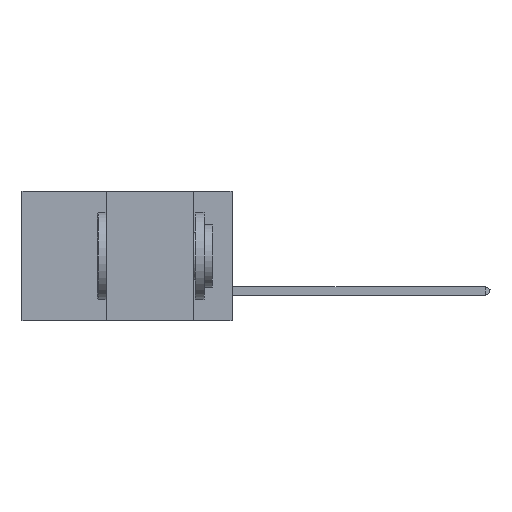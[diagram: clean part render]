
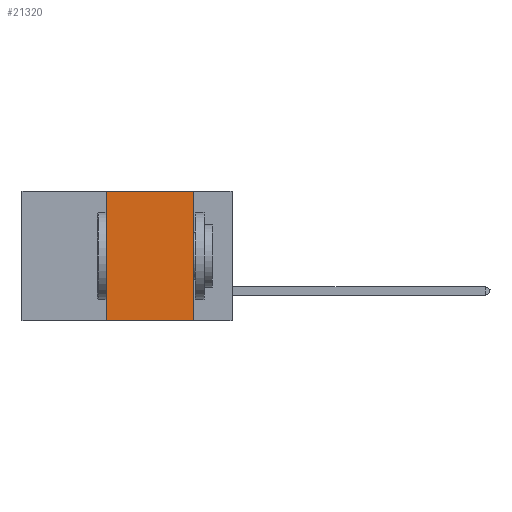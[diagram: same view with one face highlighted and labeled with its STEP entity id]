
A CAD part, left-side view. The second image highlights one B-rep face of the part: STEP entity #21320.
In plain terms, the highlighted planar face has unit normal (-1, 0, 0).
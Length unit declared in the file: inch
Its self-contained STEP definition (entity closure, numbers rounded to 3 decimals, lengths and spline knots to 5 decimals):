
#302 = VERTEX_POINT ( 'NONE', #35650 ) ;
#1284 = DIRECTION ( 'NONE',  ( 0., 0., -1. ) ) ;
#1719 = CARTESIAN_POINT ( 'NONE',  ( 0., 0.6, 0. ) ) ;
#3242 = CARTESIAN_POINT ( 'NONE',  ( 0., 0.36, 0. ) ) ;
#3380 = DIRECTION ( 'NONE',  ( 0., 0., 1. ) ) ;
#4338 = VECTOR ( 'NONE', #12556, 39.37008 ) ;
#4463 = EDGE_CURVE ( 'NONE', #43882, #36386, #37356, .T. ) ;
#4539 = EDGE_CURVE ( 'NONE', #10089, #36386, #13387, .T. ) ;
#4849 = CARTESIAN_POINT ( 'NONE',  ( 0., 0.11, 0. ) ) ;
#5787 = ORIENTED_EDGE ( 'NONE', *, *, #4539, .T. ) ;
#10089 = VERTEX_POINT ( 'NONE', #41635 ) ;
#10164 = EDGE_LOOP ( 'NONE', ( #34130, #27813, #40369, #5787 ) ) ;
#12556 = DIRECTION ( 'NONE',  ( 0., -1., 0. ) ) ;
#12999 = CARTESIAN_POINT ( 'NONE',  ( 0., 0.11, -0.37 ) ) ;
#13086 = LINE ( 'NONE', #3242, #29593 ) ;
#13387 = LINE ( 'NONE', #32825, #4338 ) ;
#13529 = VECTOR ( 'NONE', #14901, 39.37008 ) ;
#14901 = DIRECTION ( 'NONE',  ( 0., -1., 0. ) ) ;
#18009 = DIRECTION ( 'NONE',  ( 0., 0., -1. ) ) ;
#19290 = VECTOR ( 'NONE', #1284, 39.37008 ) ;
#20704 = PLANE ( 'NONE',  #22603 ) ;
#21320 = ADVANCED_FACE ( 'NONE', ( #31397 ), #20704, .F. ) ;
#22603 = AXIS2_PLACEMENT_3D ( 'NONE', #37785, #31460, #18009 ) ;
#27813 = ORIENTED_EDGE ( 'NONE', *, *, #36115, .F. ) ;
#29593 = VECTOR ( 'NONE', #3380, 39.37008 ) ;
#31397 = FACE_OUTER_BOUND ( 'NONE', #10164, .T. ) ;
#31460 = DIRECTION ( 'NONE',  ( 1., 0., 0. ) ) ;
#32190 = LINE ( 'NONE', #1719, #13529 ) ;
#32825 = CARTESIAN_POINT ( 'NONE',  ( 0., 0.6, -0.37 ) ) ;
#33353 = CARTESIAN_POINT ( 'NONE',  ( 0., 0.11, 0. ) ) ;
#34130 = ORIENTED_EDGE ( 'NONE', *, *, #4463, .F. ) ;
#35321 = EDGE_CURVE ( 'NONE', #10089, #302, #13086, .T. ) ;
#35650 = CARTESIAN_POINT ( 'NONE',  ( 0., 0.36, 0. ) ) ;
#36115 = EDGE_CURVE ( 'NONE', #302, #43882, #32190, .T. ) ;
#36386 = VERTEX_POINT ( 'NONE', #12999 ) ;
#37356 = LINE ( 'NONE', #4849, #19290 ) ;
#37785 = CARTESIAN_POINT ( 'NONE',  ( 0., 0.6, 0. ) ) ;
#40369 = ORIENTED_EDGE ( 'NONE', *, *, #35321, .F. ) ;
#41635 = CARTESIAN_POINT ( 'NONE',  ( 0., 0.36, -0.37 ) ) ;
#43882 = VERTEX_POINT ( 'NONE', #33353 ) ;
